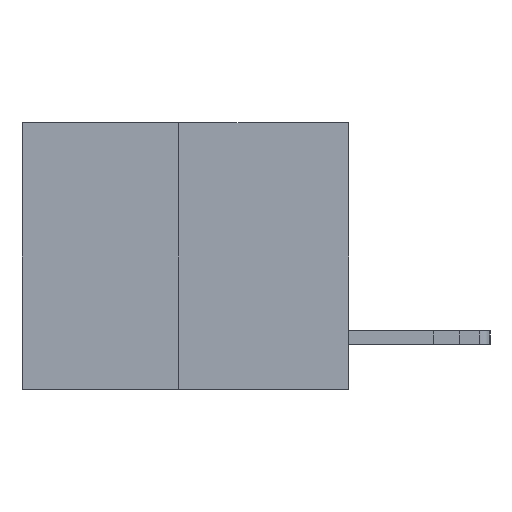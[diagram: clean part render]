
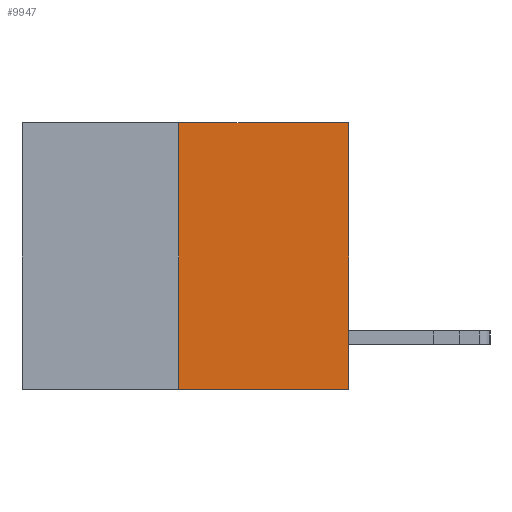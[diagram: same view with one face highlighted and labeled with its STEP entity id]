
A CAD part, left-side view. The second image highlights one B-rep face of the part: STEP entity #9947.
In plain terms, the highlighted planar face has unit normal (-1, 0, 0).
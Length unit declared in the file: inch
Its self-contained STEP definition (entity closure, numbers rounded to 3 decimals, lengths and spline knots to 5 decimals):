
#168 = VECTOR ( 'NONE', #7773, 39.37008 ) ;
#409 = LINE ( 'NONE', #1251, #8913 ) ;
#541 = EDGE_CURVE ( 'NONE', #1530, #10024, #14940, .T. ) ;
#692 = CARTESIAN_POINT ( 'NONE',  ( 0., 0., 0. ) ) ;
#1067 = CARTESIAN_POINT ( 'NONE',  ( 0., 0., -0.49 ) ) ;
#1251 = CARTESIAN_POINT ( 'NONE',  ( 0., 0.312, -0.49 ) ) ;
#1530 = VERTEX_POINT ( 'NONE', #16648 ) ;
#1656 = EDGE_CURVE ( 'NONE', #10024, #13590, #13175, .T. ) ;
#2103 = DIRECTION ( 'NONE',  ( 0., -1., 0. ) ) ;
#3205 = VERTEX_POINT ( 'NONE', #4533 ) ;
#3313 = DIRECTION ( 'NONE',  ( 0., -1., 0. ) ) ;
#3514 = EDGE_CURVE ( 'NONE', #1530, #3205, #409, .T. ) ;
#4234 = ORIENTED_EDGE ( 'NONE', *, *, #4807, .F. ) ;
#4491 = DIRECTION ( 'NONE',  ( 1., 0., 0. ) ) ;
#4533 = CARTESIAN_POINT ( 'NONE',  ( 0., 0.312, 0. ) ) ;
#4807 = EDGE_CURVE ( 'NONE', #3205, #13590, #8816, .T. ) ;
#5546 = DIRECTION ( 'NONE',  ( 0., 0., -1. ) ) ;
#6594 = ORIENTED_EDGE ( 'NONE', *, *, #3514, .F. ) ;
#7253 = DIRECTION ( 'NONE',  ( 0., 0., 1. ) ) ;
#7773 = DIRECTION ( 'NONE',  ( 0., 0., 1. ) ) ;
#7856 = ORIENTED_EDGE ( 'NONE', *, *, #1656, .T. ) ;
#8689 = CARTESIAN_POINT ( 'NONE',  ( 0., 0.6, 0. ) ) ;
#8816 = LINE ( 'NONE', #8689, #16909 ) ;
#8913 = VECTOR ( 'NONE', #7253, 39.37008 ) ;
#9116 = CARTESIAN_POINT ( 'NONE',  ( 0., 0., 0. ) ) ;
#9947 = ADVANCED_FACE ( 'NONE', ( #16844 ), #14836, .F. ) ;
#10024 = VERTEX_POINT ( 'NONE', #1067 ) ;
#11386 = VECTOR ( 'NONE', #2103, 39.37008 ) ;
#11631 = ORIENTED_EDGE ( 'NONE', *, *, #541, .T. ) ;
#12002 = AXIS2_PLACEMENT_3D ( 'NONE', #12366, #4491, #5546 ) ;
#12255 = EDGE_LOOP ( 'NONE', ( #6594, #11631, #7856, #4234 ) ) ;
#12366 = CARTESIAN_POINT ( 'NONE',  ( 0., 0.6, 0. ) ) ;
#13175 = LINE ( 'NONE', #9116, #168 ) ;
#13590 = VERTEX_POINT ( 'NONE', #692 ) ;
#14836 = PLANE ( 'NONE',  #12002 ) ;
#14940 = LINE ( 'NONE', #15148, #11386 ) ;
#15148 = CARTESIAN_POINT ( 'NONE',  ( 0., 0.6, -0.49 ) ) ;
#16648 = CARTESIAN_POINT ( 'NONE',  ( 0., 0.312, -0.49 ) ) ;
#16844 = FACE_OUTER_BOUND ( 'NONE', #12255, .T. ) ;
#16909 = VECTOR ( 'NONE', #3313, 39.37008 ) ;
